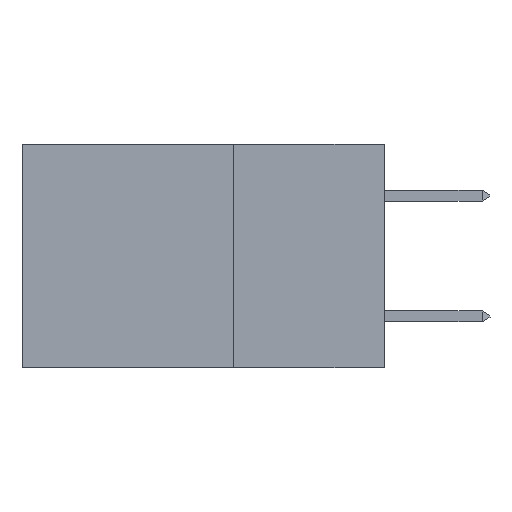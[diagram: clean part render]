
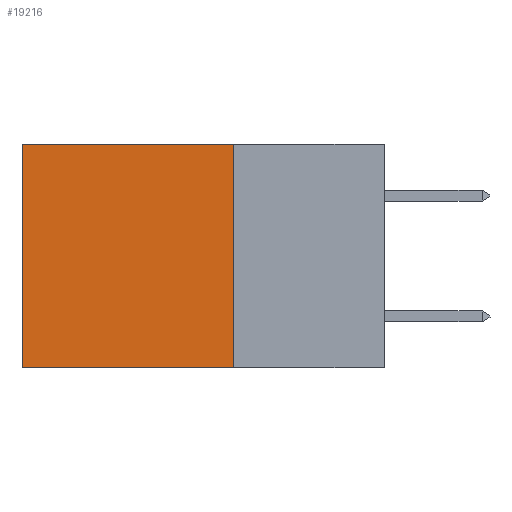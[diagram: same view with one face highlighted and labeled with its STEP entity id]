
A CAD part, left-side view. The second image highlights one B-rep face of the part: STEP entity #19216.
In plain terms, the highlighted planar face has unit normal (-1, 0, 0).
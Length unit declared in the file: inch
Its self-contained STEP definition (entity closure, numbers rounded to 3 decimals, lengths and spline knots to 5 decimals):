
#147 = LINE ( 'NONE', #13527, #20319 ) ;
#578 = ORIENTED_EDGE ( 'NONE', *, *, #13123, .T. ) ;
#1061 = AXIS2_PLACEMENT_3D ( 'NONE', #12940, #15991, #6806 ) ;
#1073 = EDGE_LOOP ( 'NONE', ( #578, #18824, #16430, #4339 ) ) ;
#2122 = CARTESIAN_POINT ( 'NONE',  ( 0.2875, 0.25, -0.37 ) ) ;
#2684 = VECTOR ( 'NONE', #3827, 39.37008 ) ;
#3733 = CARTESIAN_POINT ( 'NONE',  ( 0.2875, 0.25, 0. ) ) ;
#3827 = DIRECTION ( 'NONE',  ( 0., 1., 0. ) ) ;
#3828 = CARTESIAN_POINT ( 'NONE',  ( 0.2875, 0.6, 0. ) ) ;
#4339 = ORIENTED_EDGE ( 'NONE', *, *, #19901, .T. ) ;
#5285 = VERTEX_POINT ( 'NONE', #12132 ) ;
#6366 = VERTEX_POINT ( 'NONE', #3733 ) ;
#6806 = DIRECTION ( 'NONE',  ( 0., 0., -1. ) ) ;
#7602 = EDGE_CURVE ( 'NONE', #5285, #9974, #10618, .T. ) ;
#8714 = DIRECTION ( 'NONE',  ( 0., 1., 0. ) ) ;
#8863 = DIRECTION ( 'NONE',  ( 0., 0., -1. ) ) ;
#9192 = LINE ( 'NONE', #13051, #12814 ) ;
#9821 = PLANE ( 'NONE',  #1061 ) ;
#9974 = VERTEX_POINT ( 'NONE', #17595 ) ;
#10618 = LINE ( 'NONE', #2122, #2684 ) ;
#12132 = CARTESIAN_POINT ( 'NONE',  ( 0.2875, 0.25, -0.37 ) ) ;
#12814 = VECTOR ( 'NONE', #8714, 39.37008 ) ;
#12940 = CARTESIAN_POINT ( 'NONE',  ( 0.2875, 0.25, 0. ) ) ;
#13051 = CARTESIAN_POINT ( 'NONE',  ( 0.2875, 0.25, 0. ) ) ;
#13123 = EDGE_CURVE ( 'NONE', #16071, #9974, #13684, .T. ) ;
#13527 = CARTESIAN_POINT ( 'NONE',  ( 0.2875, 0.25, 0. ) ) ;
#13684 = LINE ( 'NONE', #3828, #18292 ) ;
#14704 = DIRECTION ( 'NONE',  ( 0., 0., -1. ) ) ;
#15724 = CARTESIAN_POINT ( 'NONE',  ( 0.2875, 0.6, 0. ) ) ;
#15991 = DIRECTION ( 'NONE',  ( 1., 0., 0. ) ) ;
#16071 = VERTEX_POINT ( 'NONE', #15724 ) ;
#16413 = EDGE_CURVE ( 'NONE', #6366, #5285, #147, .T. ) ;
#16430 = ORIENTED_EDGE ( 'NONE', *, *, #16413, .F. ) ;
#17595 = CARTESIAN_POINT ( 'NONE',  ( 0.2875, 0.6, -0.37 ) ) ;
#17635 = FACE_OUTER_BOUND ( 'NONE', #1073, .T. ) ;
#18292 = VECTOR ( 'NONE', #14704, 39.37008 ) ;
#18824 = ORIENTED_EDGE ( 'NONE', *, *, #7602, .F. ) ;
#19216 = ADVANCED_FACE ( 'NONE', ( #17635 ), #9821, .F. ) ;
#19901 = EDGE_CURVE ( 'NONE', #6366, #16071, #9192, .T. ) ;
#20319 = VECTOR ( 'NONE', #8863, 39.37008 ) ;
